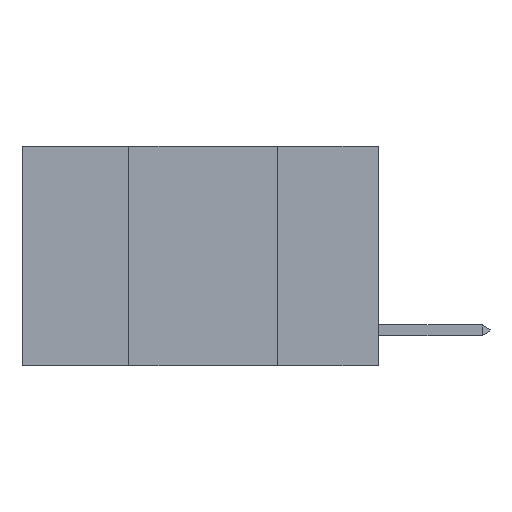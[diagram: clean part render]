
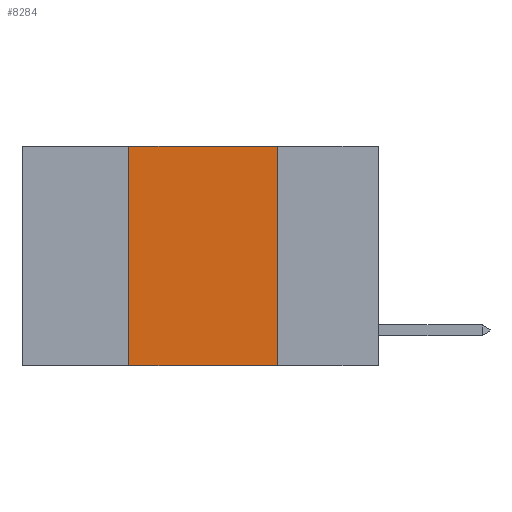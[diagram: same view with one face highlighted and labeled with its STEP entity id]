
A CAD part, left-side view. The second image highlights one B-rep face of the part: STEP entity #8284.
In plain terms, the highlighted planar face has unit normal (-1, 0, 0).
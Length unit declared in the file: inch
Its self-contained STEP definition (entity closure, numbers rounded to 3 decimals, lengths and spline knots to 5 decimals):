
#102 = PLANE ( 'NONE',  #6462 ) ;
#1577 = EDGE_LOOP ( 'NONE', ( #6232, #13651, #8982, #11209 ) ) ;
#2265 = VECTOR ( 'NONE', #8852, 39.37008 ) ;
#2321 = CARTESIAN_POINT ( 'NONE',  ( 0., 0.42, 0. ) ) ;
#2414 = DIRECTION ( 'NONE',  ( 1., 0., 0. ) ) ;
#2603 = VERTEX_POINT ( 'NONE', #2321 ) ;
#2646 = CARTESIAN_POINT ( 'NONE',  ( 0., 0.6, 0. ) ) ;
#3153 = CARTESIAN_POINT ( 'NONE',  ( 0., 0.6, 0. ) ) ;
#3759 = DIRECTION ( 'NONE',  ( 0., 0., -1. ) ) ;
#3819 = CARTESIAN_POINT ( 'NONE',  ( 0., 0.42, -0.37 ) ) ;
#3935 = VERTEX_POINT ( 'NONE', #6845 ) ;
#4910 = EDGE_CURVE ( 'NONE', #2603, #7976, #14576, .T. ) ;
#4911 = CARTESIAN_POINT ( 'NONE',  ( 0., 0.17, 0. ) ) ;
#5352 = EDGE_CURVE ( 'NONE', #11588, #3935, #7868, .T. ) ;
#6232 = ORIENTED_EDGE ( 'NONE', *, *, #13893, .F. ) ;
#6462 = AXIS2_PLACEMENT_3D ( 'NONE', #2646, #2414, #3759 ) ;
#6845 = CARTESIAN_POINT ( 'NONE',  ( 0., 0.17, -0.37 ) ) ;
#7426 = EDGE_CURVE ( 'NONE', #11588, #2603, #13535, .T. ) ;
#7868 = LINE ( 'NONE', #10114, #9610 ) ;
#7869 = DIRECTION ( 'NONE',  ( 0., 0., 1. ) ) ;
#7976 = VERTEX_POINT ( 'NONE', #14007 ) ;
#8284 = ADVANCED_FACE ( 'NONE', ( #9170 ), #102, .F. ) ;
#8852 = DIRECTION ( 'NONE',  ( 0., -1., 0. ) ) ;
#8917 = CARTESIAN_POINT ( 'NONE',  ( 0., 0.42, 0. ) ) ;
#8982 = ORIENTED_EDGE ( 'NONE', *, *, #7426, .F. ) ;
#9170 = FACE_OUTER_BOUND ( 'NONE', #1577, .T. ) ;
#9610 = VECTOR ( 'NONE', #11220, 39.37008 ) ;
#10114 = CARTESIAN_POINT ( 'NONE',  ( 0., 0.6, -0.37 ) ) ;
#10346 = VECTOR ( 'NONE', #13979, 39.37008 ) ;
#10577 = LINE ( 'NONE', #4911, #10346 ) ;
#11132 = VECTOR ( 'NONE', #7869, 39.37008 ) ;
#11209 = ORIENTED_EDGE ( 'NONE', *, *, #5352, .T. ) ;
#11220 = DIRECTION ( 'NONE',  ( 0., -1., 0. ) ) ;
#11588 = VERTEX_POINT ( 'NONE', #3819 ) ;
#13535 = LINE ( 'NONE', #8917, #11132 ) ;
#13651 = ORIENTED_EDGE ( 'NONE', *, *, #4910, .F. ) ;
#13893 = EDGE_CURVE ( 'NONE', #7976, #3935, #10577, .T. ) ;
#13979 = DIRECTION ( 'NONE',  ( 0., 0., -1. ) ) ;
#14007 = CARTESIAN_POINT ( 'NONE',  ( 0., 0.17, 0. ) ) ;
#14576 = LINE ( 'NONE', #3153, #2265 ) ;
